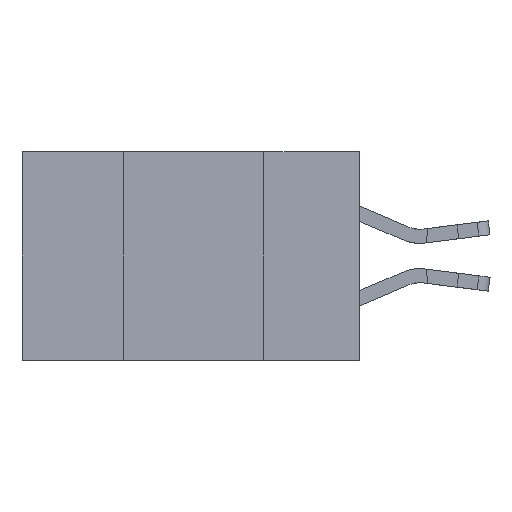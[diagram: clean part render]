
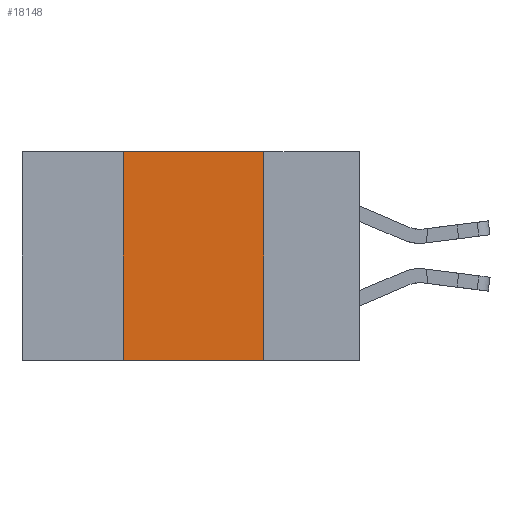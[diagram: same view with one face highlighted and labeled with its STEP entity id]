
A CAD part, left-side view. The second image highlights one B-rep face of the part: STEP entity #18148.
In plain terms, the highlighted planar face has unit normal (-1, 0, 0).
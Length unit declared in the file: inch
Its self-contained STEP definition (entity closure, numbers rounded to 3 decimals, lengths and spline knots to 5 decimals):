
#16 = CARTESIAN_POINT ( 'NONE',  ( 0., 0.42, 0. ) ) ;
#97 = EDGE_CURVE ( 'NONE', #2062, #13511, #9147, .T. ) ;
#1371 = LINE ( 'NONE', #29087, #9923 ) ;
#1901 = CARTESIAN_POINT ( 'NONE',  ( 0., 0.6, 0. ) ) ;
#2062 = VERTEX_POINT ( 'NONE', #16 ) ;
#2757 = CARTESIAN_POINT ( 'NONE',  ( 0., 0.42, 0. ) ) ;
#2800 = PLANE ( 'NONE',  #12937 ) ;
#3376 = LINE ( 'NONE', #27611, #24579 ) ;
#3396 = CARTESIAN_POINT ( 'NONE',  ( 0., 0.17, 0. ) ) ;
#6383 = EDGE_CURVE ( 'NONE', #22766, #29720, #3376, .T. ) ;
#6680 = VECTOR ( 'NONE', #10041, 39.37008 ) ;
#8823 = CARTESIAN_POINT ( 'NONE',  ( 0., 0.42, -0.37 ) ) ;
#9147 = LINE ( 'NONE', #1901, #26605 ) ;
#9923 = VECTOR ( 'NONE', #27418, 39.37008 ) ;
#10041 = DIRECTION ( 'NONE',  ( 0., 0., 1. ) ) ;
#11502 = DIRECTION ( 'NONE',  ( 0., -1., 0. ) ) ;
#12937 = AXIS2_PLACEMENT_3D ( 'NONE', #19836, #19426, #29207 ) ;
#13511 = VERTEX_POINT ( 'NONE', #3396 ) ;
#14993 = EDGE_CURVE ( 'NONE', #13511, #29720, #1371, .T. ) ;
#15498 = EDGE_LOOP ( 'NONE', ( #22878, #27493, #27978, #20696 ) ) ;
#17932 = FACE_OUTER_BOUND ( 'NONE', #15498, .T. ) ;
#18148 = ADVANCED_FACE ( 'NONE', ( #17932 ), #2800, .F. ) ;
#18251 = DIRECTION ( 'NONE',  ( 0., -1., 0. ) ) ;
#19287 = LINE ( 'NONE', #2757, #6680 ) ;
#19426 = DIRECTION ( 'NONE',  ( 1., 0., 0. ) ) ;
#19836 = CARTESIAN_POINT ( 'NONE',  ( 0., 0.6, 0. ) ) ;
#20256 = EDGE_CURVE ( 'NONE', #22766, #2062, #19287, .T. ) ;
#20696 = ORIENTED_EDGE ( 'NONE', *, *, #6383, .T. ) ;
#22766 = VERTEX_POINT ( 'NONE', #8823 ) ;
#22878 = ORIENTED_EDGE ( 'NONE', *, *, #14993, .F. ) ;
#24579 = VECTOR ( 'NONE', #18251, 39.37008 ) ;
#26605 = VECTOR ( 'NONE', #11502, 39.37008 ) ;
#27343 = CARTESIAN_POINT ( 'NONE',  ( 0., 0.17, -0.37 ) ) ;
#27418 = DIRECTION ( 'NONE',  ( 0., 0., -1. ) ) ;
#27493 = ORIENTED_EDGE ( 'NONE', *, *, #97, .F. ) ;
#27611 = CARTESIAN_POINT ( 'NONE',  ( 0., 0.6, -0.37 ) ) ;
#27978 = ORIENTED_EDGE ( 'NONE', *, *, #20256, .F. ) ;
#29087 = CARTESIAN_POINT ( 'NONE',  ( 0., 0.17, 0. ) ) ;
#29207 = DIRECTION ( 'NONE',  ( 0., 0., -1. ) ) ;
#29720 = VERTEX_POINT ( 'NONE', #27343 ) ;
